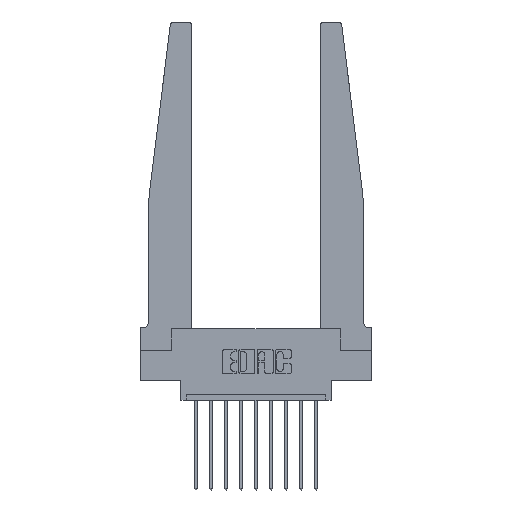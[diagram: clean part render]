
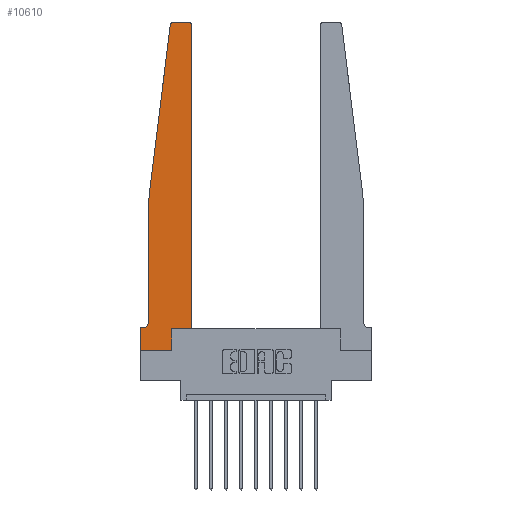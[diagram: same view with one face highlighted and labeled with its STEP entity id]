
A CAD part, top view. The second image highlights one B-rep face of the part: STEP entity #10610.
In plain terms, the highlighted planar face has unit normal (0, 0, 1).
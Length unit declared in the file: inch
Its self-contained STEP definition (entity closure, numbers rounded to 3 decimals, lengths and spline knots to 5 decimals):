
#83 = EDGE_CURVE ( 'NONE', #2367, #13360, #11653, .T. ) ;
#107 = DIRECTION ( 'NONE',  ( 1., 0., 0. ) ) ;
#170 = EDGE_CURVE ( 'NONE', #2591, #2907, #172, .T. ) ;
#172 = CIRCLE ( 'NONE', #14372, 0.05 ) ;
#334 = VECTOR ( 'NONE', #8536, 39.37008 ) ;
#883 = CARTESIAN_POINT ( 'NONE',  ( 0.015, 0.1875, 0.37 ) ) ;
#890 = ORIENTED_EDGE ( 'NONE', *, *, #8869, .T. ) ;
#1139 = AXIS2_PLACEMENT_3D ( 'NONE', #7600, #12355, #107 ) ;
#1142 = CARTESIAN_POINT ( 'NONE',  ( 0.425, 0.18, 0.37 ) ) ;
#1333 = DIRECTION ( 'NONE',  ( 0., -1., 0. ) ) ;
#1374 = VECTOR ( 'NONE', #1718, 39.37008 ) ;
#1718 = DIRECTION ( 'NONE',  ( -1., 0., 0. ) ) ;
#1745 = DIRECTION ( 'NONE',  ( 0., 0., -1. ) ) ;
#1892 = DIRECTION ( 'NONE',  ( -0.122, -0.992, 0. ) ) ;
#1926 = ORIENTED_EDGE ( 'NONE', *, *, #10451, .T. ) ;
#1948 = VERTEX_POINT ( 'NONE', #3724 ) ;
#2078 = DIRECTION ( 'NONE',  ( 1., 0., 0. ) ) ;
#2123 = LINE ( 'NONE', #4446, #13271 ) ;
#2359 = DIRECTION ( 'NONE',  ( 0., 0., 1. ) ) ;
#2367 = VERTEX_POINT ( 'NONE', #10187 ) ;
#2542 = CARTESIAN_POINT ( 'NONE',  ( 0.2605, 0.18, 0.37 ) ) ;
#2591 = VERTEX_POINT ( 'NONE', #9631 ) ;
#2771 = ORIENTED_EDGE ( 'NONE', *, *, #13600, .T. ) ;
#2907 = VERTEX_POINT ( 'NONE', #883 ) ;
#3047 = AXIS2_PLACEMENT_3D ( 'NONE', #13954, #10598, #11764 ) ;
#3083 = CARTESIAN_POINT ( 'NONE',  ( 0.395, 2.72, 0.37 ) ) ;
#3588 = CARTESIAN_POINT ( 'NONE',  ( 0.2605, 0.18, 0.37 ) ) ;
#3665 = CARTESIAN_POINT ( 'NONE',  ( 0.065, 1.25, 0.37 ) ) ;
#3724 = CARTESIAN_POINT ( 'NONE',  ( 0., 0.1875, 0.37 ) ) ;
#3804 = ORIENTED_EDGE ( 'NONE', *, *, #83, .T. ) ;
#4046 = CARTESIAN_POINT ( 'NONE',  ( 0.065, 0.1875, 0.37 ) ) ;
#4255 = LINE ( 'NONE', #10324, #12378 ) ;
#4374 = VECTOR ( 'NONE', #12971, 39.37008 ) ;
#4437 = CARTESIAN_POINT ( 'NONE',  ( 0.24675, 2.72367, 0.37 ) ) ;
#4446 = CARTESIAN_POINT ( 'NONE',  ( 0.065, 1.25, 0.37 ) ) ;
#4488 = EDGE_CURVE ( 'NONE', #7539, #5913, #9760, .T. ) ;
#4568 = DIRECTION ( 'NONE',  ( 0., 1., 0. ) ) ;
#4953 = ORIENTED_EDGE ( 'NONE', *, *, #170, .T. ) ;
#5382 = ORIENTED_EDGE ( 'NONE', *, *, #11505, .T. ) ;
#5446 = CARTESIAN_POINT ( 'NONE',  ( 0., 0., 0.37 ) ) ;
#5600 = ORIENTED_EDGE ( 'NONE', *, *, #11942, .T. ) ;
#5637 = VERTEX_POINT ( 'NONE', #7095 ) ;
#5913 = VERTEX_POINT ( 'NONE', #4437 ) ;
#6401 = CIRCLE ( 'NONE', #15080, 0.03 ) ;
#6720 = VECTOR ( 'NONE', #4568, 39.37008 ) ;
#7095 = CARTESIAN_POINT ( 'NONE',  ( 0., 0., 0.37 ) ) ;
#7205 = LINE ( 'NONE', #1142, #4374 ) ;
#7216 = DIRECTION ( 'NONE',  ( -1., 0., 0. ) ) ;
#7327 = EDGE_CURVE ( 'NONE', #5913, #12291, #2123, .T. ) ;
#7336 = VECTOR ( 'NONE', #8950, 39.37008 ) ;
#7395 = LINE ( 'NONE', #3665, #11851 ) ;
#7516 = FACE_OUTER_BOUND ( 'NONE', #9614, .T. ) ;
#7539 = VERTEX_POINT ( 'NONE', #8405 ) ;
#7600 = CARTESIAN_POINT ( 'NONE',  ( 0., 0.1875, 0.37 ) ) ;
#7851 = ORIENTED_EDGE ( 'NONE', *, *, #9212, .T. ) ;
#7870 = VERTEX_POINT ( 'NONE', #8011 ) ;
#8011 = CARTESIAN_POINT ( 'NONE',  ( 0.395, 2.75, 0.37 ) ) ;
#8137 = EDGE_CURVE ( 'NONE', #15248, #13551, #8463, .T. ) ;
#8405 = CARTESIAN_POINT ( 'NONE',  ( 0.27653, 2.75, 0.37 ) ) ;
#8439 = CARTESIAN_POINT ( 'NONE',  ( 0.425, 0.18, 0.37 ) ) ;
#8463 = LINE ( 'NONE', #2542, #334 ) ;
#8536 = DIRECTION ( 'NONE',  ( 0., 1., 0. ) ) ;
#8869 = EDGE_CURVE ( 'NONE', #2907, #1948, #11135, .T. ) ;
#8950 = DIRECTION ( 'NONE',  ( 0., -1., 0. ) ) ;
#9044 = ORIENTED_EDGE ( 'NONE', *, *, #10347, .T. ) ;
#9212 = EDGE_CURVE ( 'NONE', #7870, #7539, #10572, .T. ) ;
#9305 = ORIENTED_EDGE ( 'NONE', *, *, #7327, .T. ) ;
#9614 = EDGE_LOOP ( 'NONE', ( #7851, #13842, #9305, #5382, #4953, #890, #9044, #5600, #13112, #1926, #3804, #2771 ) ) ;
#9631 = CARTESIAN_POINT ( 'NONE',  ( 0.065, 0.2375, 0.37 ) ) ;
#9760 = CIRCLE ( 'NONE', #3047, 0.03 ) ;
#10187 = CARTESIAN_POINT ( 'NONE',  ( 0.425, 0.18, 0.37 ) ) ;
#10324 = CARTESIAN_POINT ( 'NONE',  ( 0., 0., 0.37 ) ) ;
#10347 = EDGE_CURVE ( 'NONE', #1948, #5637, #13456, .T. ) ;
#10451 = EDGE_CURVE ( 'NONE', #13551, #2367, #7205, .T. ) ;
#10572 = LINE ( 'NONE', #15374, #14295 ) ;
#10598 = DIRECTION ( 'NONE',  ( 0., 0., 1. ) ) ;
#10610 = ADVANCED_FACE ( 'NONE', ( #7516 ), #10937, .T. ) ;
#10720 = CARTESIAN_POINT ( 'NONE',  ( 0.425, 2.72, 0.37 ) ) ;
#10937 = PLANE ( 'NONE',  #1139 ) ;
#11135 = LINE ( 'NONE', #4046, #1374 ) ;
#11505 = EDGE_CURVE ( 'NONE', #12291, #2591, #7395, .T. ) ;
#11653 = LINE ( 'NONE', #8439, #6720 ) ;
#11764 = DIRECTION ( 'NONE',  ( 1., 0., 0. ) ) ;
#11851 = VECTOR ( 'NONE', #1333, 39.37008 ) ;
#11942 = EDGE_CURVE ( 'NONE', #5637, #15248, #4255, .T. ) ;
#12256 = CARTESIAN_POINT ( 'NONE',  ( 0.015, 0.2375, 0.37 ) ) ;
#12291 = VERTEX_POINT ( 'NONE', #14583 ) ;
#12355 = DIRECTION ( 'NONE',  ( 0., 0., 1. ) ) ;
#12378 = VECTOR ( 'NONE', #2078, 39.37008 ) ;
#12971 = DIRECTION ( 'NONE',  ( 1., 0., 0. ) ) ;
#13112 = ORIENTED_EDGE ( 'NONE', *, *, #8137, .T. ) ;
#13271 = VECTOR ( 'NONE', #1892, 39.37008 ) ;
#13360 = VERTEX_POINT ( 'NONE', #10720 ) ;
#13456 = LINE ( 'NONE', #5446, #7336 ) ;
#13551 = VERTEX_POINT ( 'NONE', #3588 ) ;
#13581 = CARTESIAN_POINT ( 'NONE',  ( 0.2605, 0., 0.37 ) ) ;
#13600 = EDGE_CURVE ( 'NONE', #13360, #7870, #6401, .T. ) ;
#13842 = ORIENTED_EDGE ( 'NONE', *, *, #4488, .T. ) ;
#13954 = CARTESIAN_POINT ( 'NONE',  ( 0.27653, 2.72, 0.37 ) ) ;
#14295 = VECTOR ( 'NONE', #7216, 39.37008 ) ;
#14372 = AXIS2_PLACEMENT_3D ( 'NONE', #12256, #1745, #14506 ) ;
#14506 = DIRECTION ( 'NONE',  ( -1., 0., 0. ) ) ;
#14583 = CARTESIAN_POINT ( 'NONE',  ( 0.065, 1.25, 0.37 ) ) ;
#15080 = AXIS2_PLACEMENT_3D ( 'NONE', #3083, #2359, #15332 ) ;
#15248 = VERTEX_POINT ( 'NONE', #13581 ) ;
#15332 = DIRECTION ( 'NONE',  ( 1., 0., 0. ) ) ;
#15374 = CARTESIAN_POINT ( 'NONE',  ( 0.25, 2.75, 0.37 ) ) ;
